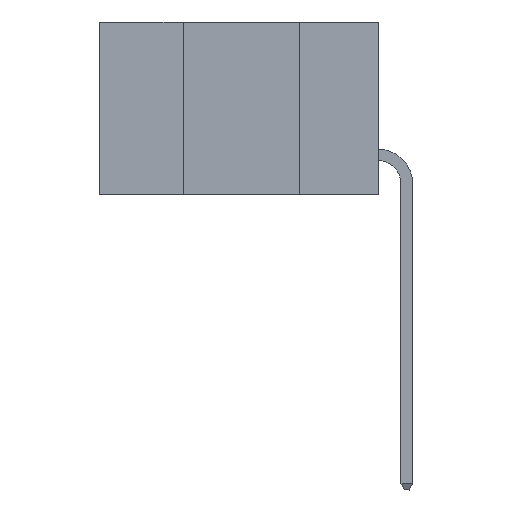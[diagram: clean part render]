
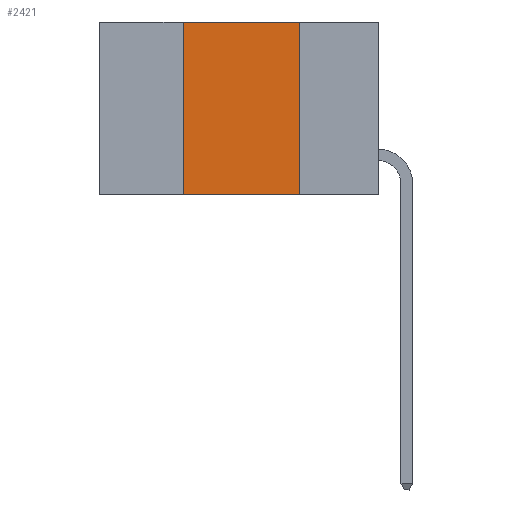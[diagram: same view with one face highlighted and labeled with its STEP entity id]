
A CAD part, left-side view. The second image highlights one B-rep face of the part: STEP entity #2421.
In plain terms, the highlighted planar face has unit normal (-1, 0, 0).
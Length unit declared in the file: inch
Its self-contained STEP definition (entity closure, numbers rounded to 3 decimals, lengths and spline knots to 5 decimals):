
#417 = VECTOR ( 'NONE', #15219, 39.37008 ) ;
#772 = AXIS2_PLACEMENT_3D ( 'NONE', #10153, #14879, #5514 ) ;
#1456 = CARTESIAN_POINT ( 'NONE',  ( 0., 0.17, 0. ) ) ;
#1715 = PLANE ( 'NONE',  #772 ) ;
#1820 = LINE ( 'NONE', #10112, #14317 ) ;
#1953 = DIRECTION ( 'NONE',  ( 0., -1., 0. ) ) ;
#2115 = CARTESIAN_POINT ( 'NONE',  ( 0., 0.6, 0. ) ) ;
#2421 = ADVANCED_FACE ( 'NONE', ( #7621 ), #1715, .F. ) ;
#3037 = LINE ( 'NONE', #9955, #15089 ) ;
#4585 = CARTESIAN_POINT ( 'NONE',  ( 0., 0.42, -0.37 ) ) ;
#4594 = LINE ( 'NONE', #11417, #11817 ) ;
#4863 = ORIENTED_EDGE ( 'NONE', *, *, #6305, .F. ) ;
#5514 = DIRECTION ( 'NONE',  ( 0., 0., -1. ) ) ;
#5956 = ORIENTED_EDGE ( 'NONE', *, *, #11744, .F. ) ;
#6305 = EDGE_CURVE ( 'NONE', #7680, #11778, #1820, .T. ) ;
#7621 = FACE_OUTER_BOUND ( 'NONE', #8381, .T. ) ;
#7680 = VERTEX_POINT ( 'NONE', #4585 ) ;
#8174 = VERTEX_POINT ( 'NONE', #1456 ) ;
#8381 = EDGE_LOOP ( 'NONE', ( #5956, #10611, #4863, #9358 ) ) ;
#9358 = ORIENTED_EDGE ( 'NONE', *, *, #14612, .T. ) ;
#9955 = CARTESIAN_POINT ( 'NONE',  ( 0., 0.6, -0.37 ) ) ;
#10112 = CARTESIAN_POINT ( 'NONE',  ( 0., 0.42, -0.37 ) ) ;
#10153 = CARTESIAN_POINT ( 'NONE',  ( 0., 0.6, 0. ) ) ;
#10341 = LINE ( 'NONE', #2115, #417 ) ;
#10413 = DIRECTION ( 'NONE',  ( 0., 0., -1. ) ) ;
#10611 = ORIENTED_EDGE ( 'NONE', *, *, #10740, .F. ) ;
#10709 = CARTESIAN_POINT ( 'NONE',  ( 0., 0.17, -0.37 ) ) ;
#10740 = EDGE_CURVE ( 'NONE', #11778, #8174, #10341, .T. ) ;
#11351 = DIRECTION ( 'NONE',  ( 0., 0., 1. ) ) ;
#11417 = CARTESIAN_POINT ( 'NONE',  ( 0., 0.17, -0.37 ) ) ;
#11744 = EDGE_CURVE ( 'NONE', #8174, #13531, #4594, .T. ) ;
#11778 = VERTEX_POINT ( 'NONE', #14903 ) ;
#11817 = VECTOR ( 'NONE', #10413, 39.37008 ) ;
#13531 = VERTEX_POINT ( 'NONE', #10709 ) ;
#14317 = VECTOR ( 'NONE', #11351, 39.37008 ) ;
#14612 = EDGE_CURVE ( 'NONE', #7680, #13531, #3037, .T. ) ;
#14879 = DIRECTION ( 'NONE',  ( 1., 0., 0. ) ) ;
#14903 = CARTESIAN_POINT ( 'NONE',  ( 0., 0.42, 0. ) ) ;
#15089 = VECTOR ( 'NONE', #1953, 39.37008 ) ;
#15219 = DIRECTION ( 'NONE',  ( 0., -1., 0. ) ) ;
